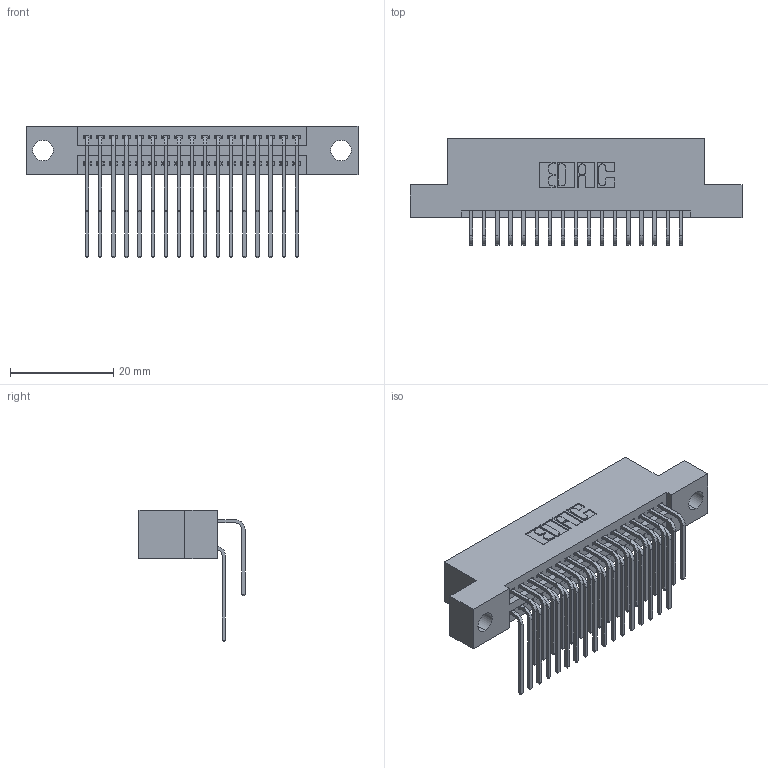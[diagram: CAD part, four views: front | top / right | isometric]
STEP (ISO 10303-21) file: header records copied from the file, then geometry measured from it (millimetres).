
FILE_DESCRIPTION (( 'STEP AP203' ), '1' );
FILE_NAME ('395-034-559-204.STEP', '2018-11-13T10:38:20', ( '' ), ( '' ), 'SwSTEP 2.0', 'SolidWorks 2016', '' );
FILE_SCHEMA (( 'CONFIG_CONTROL_DESIGN' ));
Length unit declared in the file: inch
Products named in the file (4): 345 Part_Flush Mounting Lugs - 0.156 Dia-TH; 345-292-001_559 Tail - 2; 395-034-559-204; 345-292-001_558 559 Tail - 1
Assembly tree (35 placements, depth 2):
  395-034-559-204
    345 Part_Flush Mounting Lugs - 0.156 Dia-TH
    345-292-001_558 559 Tail - 1  x17
    345-292-001_559 Tail - 2  x17
Bounding box: 64.39 x 20.56 x 25.53 mm (x, y, z)
Volume: 6131 mm3; surface area: 9316 mm2
Topology: 35 solids, 35 shells, 1894 faces, 5611 edges, 3694 vertices
Faces by surface type: plane 1270, cylinder 624
Entity records: 18359 total; most frequent: CARTESIAN_POINT 3147, ORIENTED_EDGE 3030, DIRECTION 2779, EDGE_CURVE 1515, VECTOR 1275, LINE 1275, VERTEX_POINT 1006, AXIS2_PLACEMENT_3D 752
